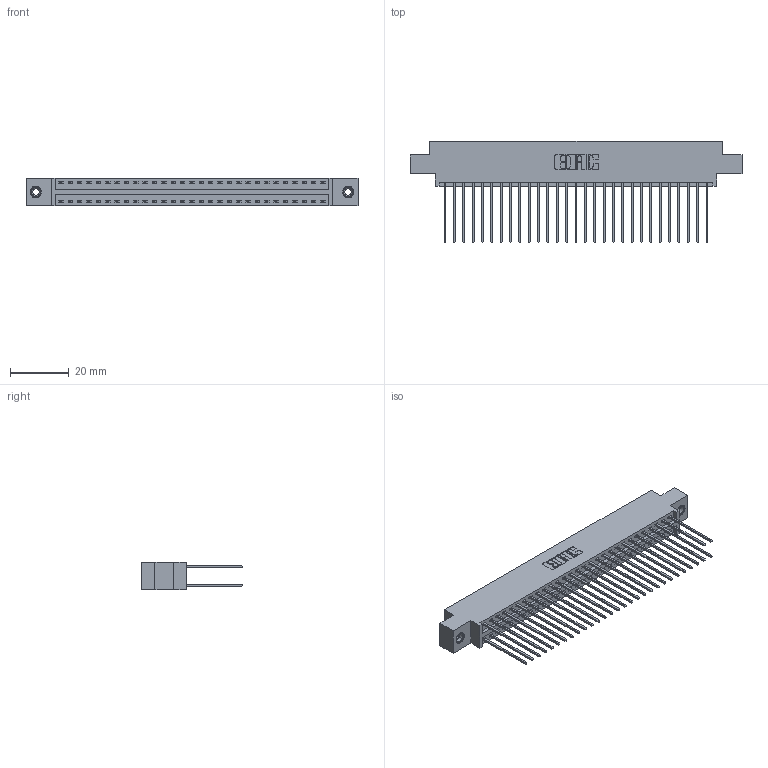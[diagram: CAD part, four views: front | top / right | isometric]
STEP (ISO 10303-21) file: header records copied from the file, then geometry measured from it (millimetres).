
FILE_DESCRIPTION (( 'STEP AP203' ), '1' );
FILE_NAME ('396-058-541-808.STEP', '2019-11-02T08:43:12', ( '' ), ( '' ), 'SwSTEP 2.0', 'SolidWorks 2016', '' );
FILE_SCHEMA (( 'CONFIG_CONTROL_DESIGN' ));
Length unit declared in the file: inch
Products named in the file (4): 345-250-001_345-250-003-102; 396-058-541-808; 346 Part_0.170 Offset - 0.156 Dia-TI; 345-292-001_345-293-141
Assembly tree (61 placements, depth 2):
  396-058-541-808
    346 Part_0.170 Offset - 0.156 Dia-TI
    345-292-001_345-293-141  x58
    345-250-001_345-250-003-102  x2
Bounding box: 112.65 x 34.29 x 9.4 mm (x, y, z)
Volume: 11055.3 mm3; surface area: 16787.4 mm2
Topology: 61 solids, 61 shells, 3202 faces, 9467 edges, 6226 vertices
Faces by surface type: plane 2142, cylinder 1044, cone 12, torus 4
Entity records: 22012 total; most frequent: CARTESIAN_POINT 3631, ORIENTED_EDGE 3558, DIRECTION 3277, EDGE_CURVE 1779, VECTOR 1511, LINE 1511, VERTEX_POINT 1180, AXIS2_PLACEMENT_3D 883
